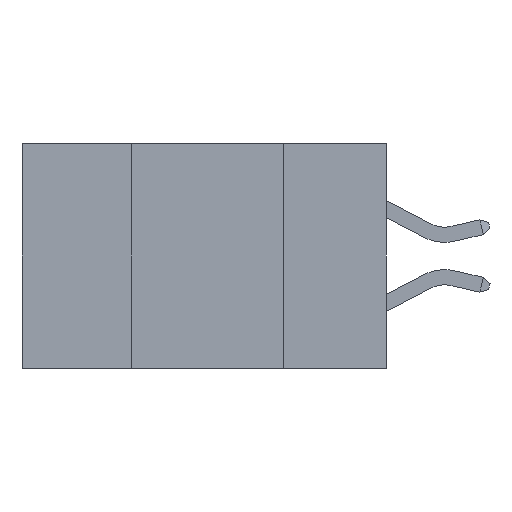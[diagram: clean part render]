
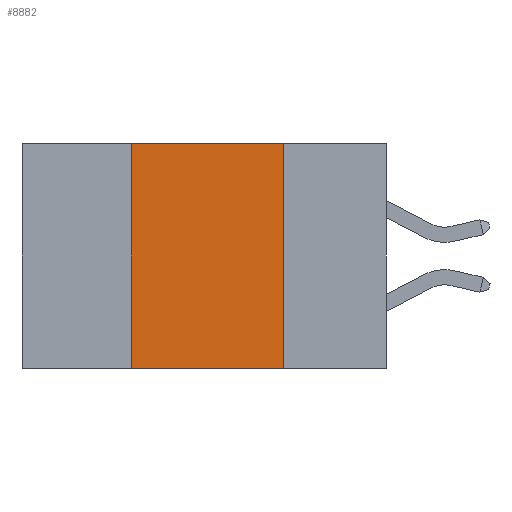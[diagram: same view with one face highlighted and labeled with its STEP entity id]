
A CAD part, left-side view. The second image highlights one B-rep face of the part: STEP entity #8882.
In plain terms, the highlighted planar face has unit normal (-1, 0, 0).
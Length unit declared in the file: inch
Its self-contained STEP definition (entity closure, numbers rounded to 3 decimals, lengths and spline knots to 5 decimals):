
#33 = CARTESIAN_POINT ( 'NONE',  ( 0., 0.42, -0.37 ) ) ;
#348 = DIRECTION ( 'NONE',  ( 1., 0., 0. ) ) ;
#1694 = CARTESIAN_POINT ( 'NONE',  ( 0., 0.6, 0. ) ) ;
#1926 = DIRECTION ( 'NONE',  ( 0., 0., -1. ) ) ;
#2207 = DIRECTION ( 'NONE',  ( 0., 0., 1. ) ) ;
#3306 = ORIENTED_EDGE ( 'NONE', *, *, #4723, .T. ) ;
#3674 = VERTEX_POINT ( 'NONE', #16290 ) ;
#3785 = CARTESIAN_POINT ( 'NONE',  ( 0., 0.42, 0. ) ) ;
#3881 = DIRECTION ( 'NONE',  ( 0., -1., 0. ) ) ;
#4723 = EDGE_CURVE ( 'NONE', #3674, #10760, #6807, .T. ) ;
#4924 = VECTOR ( 'NONE', #1926, 39.37008 ) ;
#5280 = AXIS2_PLACEMENT_3D ( 'NONE', #13412, #348, #15619 ) ;
#6113 = VECTOR ( 'NONE', #20029, 39.37008 ) ;
#6696 = VECTOR ( 'NONE', #2207, 39.37008 ) ;
#6807 = LINE ( 'NONE', #20124, #6113 ) ;
#6989 = LINE ( 'NONE', #1694, #12103 ) ;
#8882 = ADVANCED_FACE ( 'NONE', ( #21461 ), #22005, .F. ) ;
#10760 = VERTEX_POINT ( 'NONE', #19488 ) ;
#11441 = EDGE_LOOP ( 'NONE', ( #14594, #25295, #19656, #3306 ) ) ;
#11846 = CARTESIAN_POINT ( 'NONE',  ( 0., 0.17, 0. ) ) ;
#12040 = EDGE_CURVE ( 'NONE', #3674, #20579, #18270, .T. ) ;
#12103 = VECTOR ( 'NONE', #3881, 39.37008 ) ;
#13412 = CARTESIAN_POINT ( 'NONE',  ( 0., 0.6, 0. ) ) ;
#14594 = ORIENTED_EDGE ( 'NONE', *, *, #17413, .F. ) ;
#15619 = DIRECTION ( 'NONE',  ( 0., 0., -1. ) ) ;
#16290 = CARTESIAN_POINT ( 'NONE',  ( 0., 0.42, -0.37 ) ) ;
#17413 = EDGE_CURVE ( 'NONE', #17785, #10760, #22223, .T. ) ;
#17785 = VERTEX_POINT ( 'NONE', #11846 ) ;
#18071 = EDGE_CURVE ( 'NONE', #20579, #17785, #6989, .T. ) ;
#18270 = LINE ( 'NONE', #33, #6696 ) ;
#19488 = CARTESIAN_POINT ( 'NONE',  ( 0., 0.17, -0.37 ) ) ;
#19656 = ORIENTED_EDGE ( 'NONE', *, *, #12040, .F. ) ;
#20029 = DIRECTION ( 'NONE',  ( 0., -1., 0. ) ) ;
#20124 = CARTESIAN_POINT ( 'NONE',  ( 0., 0.6, -0.37 ) ) ;
#20579 = VERTEX_POINT ( 'NONE', #3785 ) ;
#21461 = FACE_OUTER_BOUND ( 'NONE', #11441, .T. ) ;
#22005 = PLANE ( 'NONE',  #5280 ) ;
#22223 = LINE ( 'NONE', #27651, #4924 ) ;
#25295 = ORIENTED_EDGE ( 'NONE', *, *, #18071, .F. ) ;
#27651 = CARTESIAN_POINT ( 'NONE',  ( 0., 0.17, -0.37 ) ) ;
